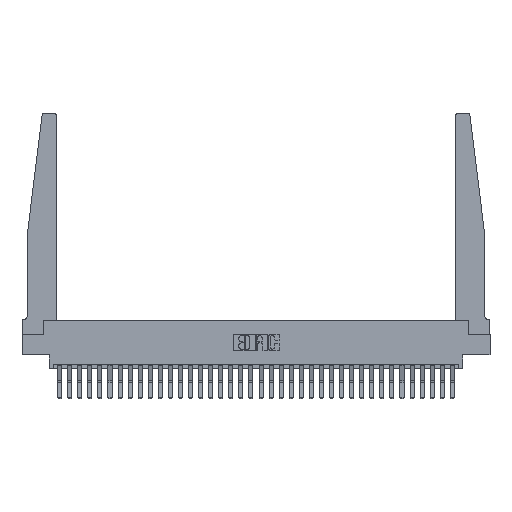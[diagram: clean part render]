
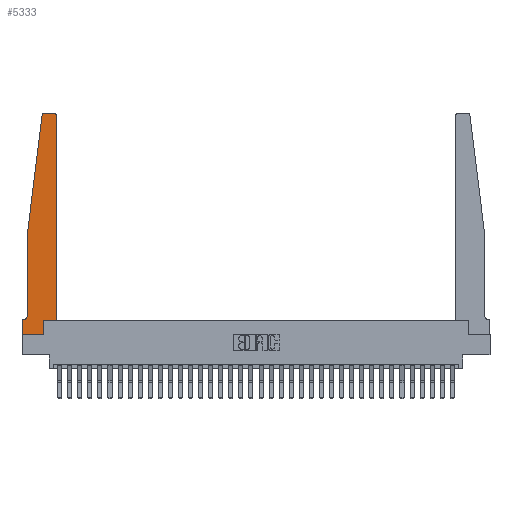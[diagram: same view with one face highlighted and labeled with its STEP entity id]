
A CAD part, top view. The second image highlights one B-rep face of the part: STEP entity #5333.
In plain terms, the highlighted planar face has unit normal (0, 0, 1).
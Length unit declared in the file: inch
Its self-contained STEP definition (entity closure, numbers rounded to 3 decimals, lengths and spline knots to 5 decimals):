
#224 = CARTESIAN_POINT ( 'NONE',  ( 0.015, 0.1875, 0.37 ) ) ;
#647 = FACE_OUTER_BOUND ( 'NONE', #2410, .T. ) ;
#749 = DIRECTION ( 'NONE',  ( -1., 0., 0. ) ) ;
#1154 = ORIENTED_EDGE ( 'NONE', *, *, #9461, .T. ) ;
#2050 = VERTEX_POINT ( 'NONE', #17733 ) ;
#2284 = CARTESIAN_POINT ( 'NONE',  ( 0.015, 0.2375, 0.37 ) ) ;
#2299 = VERTEX_POINT ( 'NONE', #224 ) ;
#2403 = VERTEX_POINT ( 'NONE', #21035 ) ;
#2410 = EDGE_LOOP ( 'NONE', ( #26028, #26406, #10843, #26067, #8552, #7177, #5358, #1154, #28891, #8631, #25623, #20784 ) ) ;
#2437 = CARTESIAN_POINT ( 'NONE',  ( 0., 0.1875, 0.37 ) ) ;
#2739 = DIRECTION ( 'NONE',  ( 0., 0., 1. ) ) ;
#2763 = DIRECTION ( 'NONE',  ( 0., 0., 1. ) ) ;
#3134 = VERTEX_POINT ( 'NONE', #16766 ) ;
#3823 = CARTESIAN_POINT ( 'NONE',  ( 0.065, 1.25, 0.37 ) ) ;
#3967 = VECTOR ( 'NONE', #10629, 39.37008 ) ;
#4483 = LINE ( 'NONE', #26536, #24884 ) ;
#4609 = EDGE_CURVE ( 'NONE', #2050, #16920, #8690, .T. ) ;
#4737 = CARTESIAN_POINT ( 'NONE',  ( 0., 0., 0.37 ) ) ;
#4884 = EDGE_CURVE ( 'NONE', #18415, #14807, #19806, .T. ) ;
#5333 = ADVANCED_FACE ( 'NONE', ( #647 ), #22418, .T. ) ;
#5358 = ORIENTED_EDGE ( 'NONE', *, *, #14366, .T. ) ;
#5405 = CARTESIAN_POINT ( 'NONE',  ( 0., 0., 0.37 ) ) ;
#5830 = VECTOR ( 'NONE', #6646, 39.37008 ) ;
#6307 = CARTESIAN_POINT ( 'NONE',  ( 0.2605, 0.18, 0.37 ) ) ;
#6414 = EDGE_CURVE ( 'NONE', #2403, #2050, #29871, .T. ) ;
#6646 = DIRECTION ( 'NONE',  ( -0.122, -0.992, 0. ) ) ;
#6795 = LINE ( 'NONE', #20847, #5830 ) ;
#7151 = LINE ( 'NONE', #4737, #17880 ) ;
#7163 = CARTESIAN_POINT ( 'NONE',  ( 0.27653, 2.75, 0.37 ) ) ;
#7177 = ORIENTED_EDGE ( 'NONE', *, *, #27318, .T. ) ;
#7199 = VECTOR ( 'NONE', #749, 39.37008 ) ;
#7926 = CARTESIAN_POINT ( 'NONE',  ( 0.2605, 0.18, 0.37 ) ) ;
#8552 = ORIENTED_EDGE ( 'NONE', *, *, #16084, .T. ) ;
#8631 = ORIENTED_EDGE ( 'NONE', *, *, #4884, .T. ) ;
#8690 = LINE ( 'NONE', #13036, #20016 ) ;
#8862 = LINE ( 'NONE', #6307, #18154 ) ;
#8898 = CIRCLE ( 'NONE', #28975, 0.03 ) ;
#9098 = VERTEX_POINT ( 'NONE', #10610 ) ;
#9461 = EDGE_CURVE ( 'NONE', #22535, #3134, #27475, .T. ) ;
#9687 = DIRECTION ( 'NONE',  ( 0., 0., -1. ) ) ;
#10459 = CARTESIAN_POINT ( 'NONE',  ( 0.27653, 2.72, 0.37 ) ) ;
#10610 = CARTESIAN_POINT ( 'NONE',  ( 0.24675, 2.72367, 0.37 ) ) ;
#10629 = DIRECTION ( 'NONE',  ( 0., 1., 0. ) ) ;
#10843 = ORIENTED_EDGE ( 'NONE', *, *, #19903, .T. ) ;
#11878 = DIRECTION ( 'NONE',  ( 0., -1., 0. ) ) ;
#12672 = CARTESIAN_POINT ( 'NONE',  ( 0.425, 0.18, 0.37 ) ) ;
#12883 = CARTESIAN_POINT ( 'NONE',  ( 0.425, 0.18, 0.37 ) ) ;
#13036 = CARTESIAN_POINT ( 'NONE',  ( 0.25, 2.75, 0.37 ) ) ;
#14366 = EDGE_CURVE ( 'NONE', #21373, #22535, #7151, .T. ) ;
#14632 = DIRECTION ( 'NONE',  ( 1., 0., 0. ) ) ;
#14807 = VERTEX_POINT ( 'NONE', #29940 ) ;
#15216 = DIRECTION ( 'NONE',  ( 1., 0., 0. ) ) ;
#15254 = CIRCLE ( 'NONE', #27079, 0.05 ) ;
#15327 = CARTESIAN_POINT ( 'NONE',  ( 0., 0.1875, 0.37 ) ) ;
#15898 = DIRECTION ( 'NONE',  ( 1., 0., 0. ) ) ;
#16084 = EDGE_CURVE ( 'NONE', #19992, #2299, #15254, .T. ) ;
#16766 = CARTESIAN_POINT ( 'NONE',  ( 0.2605, 0., 0.37 ) ) ;
#16920 = VERTEX_POINT ( 'NONE', #7163 ) ;
#17662 = EDGE_CURVE ( 'NONE', #3134, #18415, #8862, .T. ) ;
#17733 = CARTESIAN_POINT ( 'NONE',  ( 0.395, 2.75, 0.37 ) ) ;
#17880 = VECTOR ( 'NONE', #31613, 39.37008 ) ;
#18154 = VECTOR ( 'NONE', #25801, 39.37008 ) ;
#18227 = LINE ( 'NONE', #12883, #3967 ) ;
#18415 = VERTEX_POINT ( 'NONE', #7926 ) ;
#18881 = EDGE_CURVE ( 'NONE', #16920, #9098, #8898, .T. ) ;
#19806 = LINE ( 'NONE', #12672, #22050 ) ;
#19903 = EDGE_CURVE ( 'NONE', #9098, #23723, #6795, .T. ) ;
#19992 = VERTEX_POINT ( 'NONE', #26426 ) ;
#20016 = VECTOR ( 'NONE', #25453, 39.37008 ) ;
#20543 = VECTOR ( 'NONE', #15216, 39.37008 ) ;
#20556 = AXIS2_PLACEMENT_3D ( 'NONE', #15327, #2763, #22259 ) ;
#20784 = ORIENTED_EDGE ( 'NONE', *, *, #6414, .T. ) ;
#20847 = CARTESIAN_POINT ( 'NONE',  ( 0.065, 1.25, 0.37 ) ) ;
#21035 = CARTESIAN_POINT ( 'NONE',  ( 0.425, 2.72, 0.37 ) ) ;
#21373 = VERTEX_POINT ( 'NONE', #2437 ) ;
#22050 = VECTOR ( 'NONE', #14632, 39.37008 ) ;
#22259 = DIRECTION ( 'NONE',  ( 1., 0., 0. ) ) ;
#22418 = PLANE ( 'NONE',  #20556 ) ;
#22535 = VERTEX_POINT ( 'NONE', #31189 ) ;
#22972 = DIRECTION ( 'NONE',  ( 0., 0., 1. ) ) ;
#23723 = VERTEX_POINT ( 'NONE', #3823 ) ;
#24270 = EDGE_CURVE ( 'NONE', #14807, #2403, #18227, .T. ) ;
#24884 = VECTOR ( 'NONE', #11878, 39.37008 ) ;
#25239 = CARTESIAN_POINT ( 'NONE',  ( 0.395, 2.72, 0.37 ) ) ;
#25453 = DIRECTION ( 'NONE',  ( -1., 0., 0. ) ) ;
#25623 = ORIENTED_EDGE ( 'NONE', *, *, #24270, .T. ) ;
#25801 = DIRECTION ( 'NONE',  ( 0., 1., 0. ) ) ;
#26028 = ORIENTED_EDGE ( 'NONE', *, *, #4609, .T. ) ;
#26067 = ORIENTED_EDGE ( 'NONE', *, *, #30405, .T. ) ;
#26406 = ORIENTED_EDGE ( 'NONE', *, *, #18881, .T. ) ;
#26426 = CARTESIAN_POINT ( 'NONE',  ( 0.065, 0.2375, 0.37 ) ) ;
#26536 = CARTESIAN_POINT ( 'NONE',  ( 0.065, 1.25, 0.37 ) ) ;
#26776 = AXIS2_PLACEMENT_3D ( 'NONE', #25239, #22972, #15898 ) ;
#27079 = AXIS2_PLACEMENT_3D ( 'NONE', #2284, #9687, #29027 ) ;
#27318 = EDGE_CURVE ( 'NONE', #2299, #21373, #29934, .T. ) ;
#27366 = CARTESIAN_POINT ( 'NONE',  ( 0.065, 0.1875, 0.37 ) ) ;
#27475 = LINE ( 'NONE', #5405, #20543 ) ;
#28891 = ORIENTED_EDGE ( 'NONE', *, *, #17662, .T. ) ;
#28975 = AXIS2_PLACEMENT_3D ( 'NONE', #10459, #2739, #29963 ) ;
#29027 = DIRECTION ( 'NONE',  ( -1., 0., 0. ) ) ;
#29871 = CIRCLE ( 'NONE', #26776, 0.03 ) ;
#29934 = LINE ( 'NONE', #27366, #7199 ) ;
#29940 = CARTESIAN_POINT ( 'NONE',  ( 0.425, 0.18, 0.37 ) ) ;
#29963 = DIRECTION ( 'NONE',  ( 1., 0., 0. ) ) ;
#30405 = EDGE_CURVE ( 'NONE', #23723, #19992, #4483, .T. ) ;
#31189 = CARTESIAN_POINT ( 'NONE',  ( 0., 0., 0.37 ) ) ;
#31613 = DIRECTION ( 'NONE',  ( 0., -1., 0. ) ) ;
